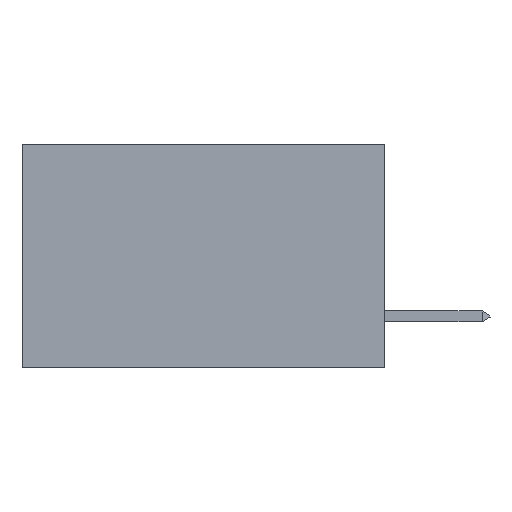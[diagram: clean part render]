
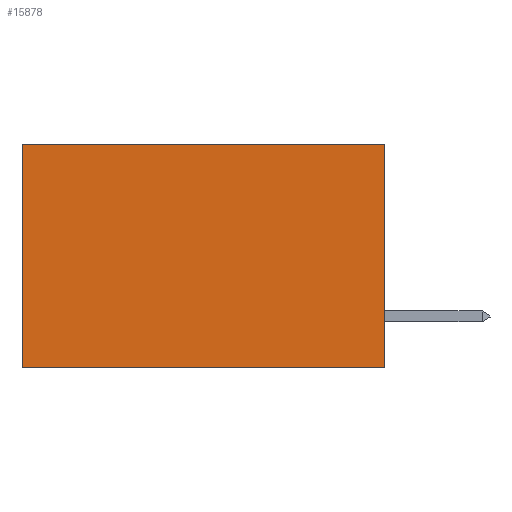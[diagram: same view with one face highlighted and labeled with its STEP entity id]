
A CAD part, left-side view. The second image highlights one B-rep face of the part: STEP entity #15878.
In plain terms, the highlighted planar face has unit normal (-1, 0, 0).
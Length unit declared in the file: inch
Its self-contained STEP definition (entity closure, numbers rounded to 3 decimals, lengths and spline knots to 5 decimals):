
#675 = FACE_OUTER_BOUND ( 'NONE', #27339, .T. ) ;
#839 = DIRECTION ( 'NONE',  ( 0., 1., 0. ) ) ;
#1555 = CARTESIAN_POINT ( 'NONE',  ( 0.2875, 0.6, 0. ) ) ;
#1616 = VECTOR ( 'NONE', #14393, 39.37008 ) ;
#1898 = CARTESIAN_POINT ( 'NONE',  ( 0.2875, 0.6, -0.37 ) ) ;
#3342 = CARTESIAN_POINT ( 'NONE',  ( 0.2875, 0., -0.37 ) ) ;
#3970 = DIRECTION ( 'NONE',  ( 1., 0., 0. ) ) ;
#4511 = LINE ( 'NONE', #24250, #13648 ) ;
#6379 = EDGE_CURVE ( 'NONE', #35337, #15375, #37589, .T. ) ;
#7239 = EDGE_CURVE ( 'NONE', #35337, #33114, #23935, .T. ) ;
#7800 = VERTEX_POINT ( 'NONE', #1898 ) ;
#8239 = EDGE_CURVE ( 'NONE', #15375, #7800, #21167, .T. ) ;
#10752 = CARTESIAN_POINT ( 'NONE',  ( 0.2875, 0., 0. ) ) ;
#11504 = CARTESIAN_POINT ( 'NONE',  ( 0.2875, 0.6, 0. ) ) ;
#11670 = CARTESIAN_POINT ( 'NONE',  ( 0.2875, 0., 0. ) ) ;
#12985 = ORIENTED_EDGE ( 'NONE', *, *, #29614, .F. ) ;
#13077 = DIRECTION ( 'NONE',  ( 0., 0., -1. ) ) ;
#13648 = VECTOR ( 'NONE', #839, 39.37008 ) ;
#13722 = PLANE ( 'NONE',  #31555 ) ;
#14393 = DIRECTION ( 'NONE',  ( 0., 0., -1. ) ) ;
#15375 = VERTEX_POINT ( 'NONE', #11504 ) ;
#15878 = ADVANCED_FACE ( 'NONE', ( #675 ), #13722, .F. ) ;
#18109 = VECTOR ( 'NONE', #33604, 39.37008 ) ;
#19087 = ORIENTED_EDGE ( 'NONE', *, *, #7239, .F. ) ;
#21167 = LINE ( 'NONE', #1555, #32013 ) ;
#22587 = ORIENTED_EDGE ( 'NONE', *, *, #8239, .T. ) ;
#23935 = LINE ( 'NONE', #11670, #1616 ) ;
#24214 = CARTESIAN_POINT ( 'NONE',  ( 0.2875, 0., 0. ) ) ;
#24250 = CARTESIAN_POINT ( 'NONE',  ( 0.2875, 0., -0.37 ) ) ;
#27339 = EDGE_LOOP ( 'NONE', ( #22587, #12985, #19087, #31222 ) ) ;
#29614 = EDGE_CURVE ( 'NONE', #33114, #7800, #4511, .T. ) ;
#30679 = DIRECTION ( 'NONE',  ( 0., 0., -1. ) ) ;
#31222 = ORIENTED_EDGE ( 'NONE', *, *, #6379, .T. ) ;
#31555 = AXIS2_PLACEMENT_3D ( 'NONE', #24214, #3970, #13077 ) ;
#31720 = CARTESIAN_POINT ( 'NONE',  ( 0.2875, 0., 0. ) ) ;
#32013 = VECTOR ( 'NONE', #30679, 39.37008 ) ;
#33114 = VERTEX_POINT ( 'NONE', #3342 ) ;
#33604 = DIRECTION ( 'NONE',  ( 0., 1., 0. ) ) ;
#35337 = VERTEX_POINT ( 'NONE', #31720 ) ;
#37589 = LINE ( 'NONE', #10752, #18109 ) ;
